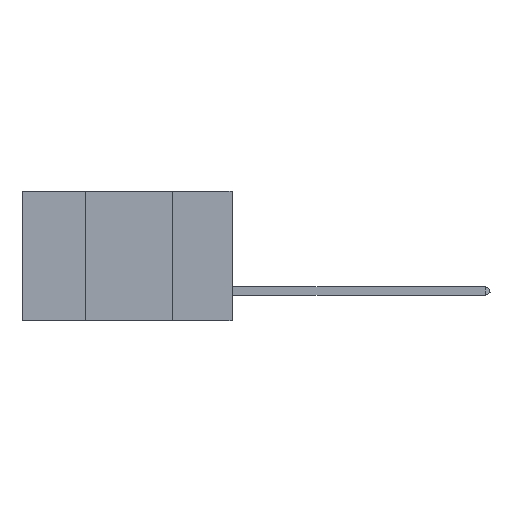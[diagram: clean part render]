
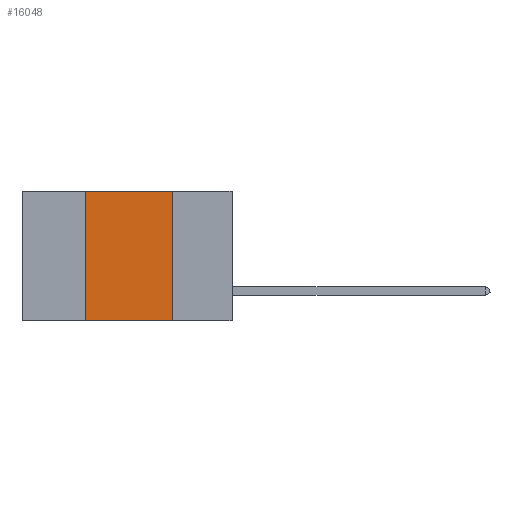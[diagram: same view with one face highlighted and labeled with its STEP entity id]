
A CAD part, left-side view. The second image highlights one B-rep face of the part: STEP entity #16048.
In plain terms, the highlighted planar face has unit normal (-1, 0, 0).
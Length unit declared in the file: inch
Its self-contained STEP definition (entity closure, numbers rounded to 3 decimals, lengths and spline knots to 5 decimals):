
#233 = EDGE_CURVE ( 'NONE', #22224, #1460, #5608, .T. ) ;
#422 = VECTOR ( 'NONE', #11954, 39.37008 ) ;
#1460 = VERTEX_POINT ( 'NONE', #13220 ) ;
#1502 = CARTESIAN_POINT ( 'NONE',  ( 0., 0.6, 0. ) ) ;
#3021 = EDGE_LOOP ( 'NONE', ( #9963, #9471, #19968, #9890 ) ) ;
#3056 = PLANE ( 'NONE',  #6564 ) ;
#3438 = LINE ( 'NONE', #16764, #9142 ) ;
#4448 = EDGE_CURVE ( 'NONE', #4482, #22224, #4647, .T. ) ;
#4482 = VERTEX_POINT ( 'NONE', #10826 ) ;
#4647 = LINE ( 'NONE', #1502, #5725 ) ;
#4759 = CARTESIAN_POINT ( 'NONE',  ( 0., 0.42, -0.37 ) ) ;
#5604 = FACE_OUTER_BOUND ( 'NONE', #3021, .T. ) ;
#5608 = LINE ( 'NONE', #22294, #422 ) ;
#5725 = VECTOR ( 'NONE', #8570, 39.37008 ) ;
#6048 = CARTESIAN_POINT ( 'NONE',  ( 0., 0.17, 0. ) ) ;
#6194 = DIRECTION ( 'NONE',  ( 0., 0., 1. ) ) ;
#6564 = AXIS2_PLACEMENT_3D ( 'NONE', #14696, #7830, #20363 ) ;
#7830 = DIRECTION ( 'NONE',  ( 1., 0., 0. ) ) ;
#8570 = DIRECTION ( 'NONE',  ( 0., -1., 0. ) ) ;
#9142 = VECTOR ( 'NONE', #6194, 39.37008 ) ;
#9471 = ORIENTED_EDGE ( 'NONE', *, *, #4448, .F. ) ;
#9890 = ORIENTED_EDGE ( 'NONE', *, *, #14965, .T. ) ;
#9963 = ORIENTED_EDGE ( 'NONE', *, *, #233, .F. ) ;
#10826 = CARTESIAN_POINT ( 'NONE',  ( 0., 0.42, 0. ) ) ;
#11089 = EDGE_CURVE ( 'NONE', #11139, #4482, #3438, .T. ) ;
#11139 = VERTEX_POINT ( 'NONE', #4759 ) ;
#11954 = DIRECTION ( 'NONE',  ( 0., 0., -1. ) ) ;
#12489 = LINE ( 'NONE', #17504, #20056 ) ;
#13220 = CARTESIAN_POINT ( 'NONE',  ( 0., 0.17, -0.37 ) ) ;
#13827 = DIRECTION ( 'NONE',  ( 0., -1., 0. ) ) ;
#14696 = CARTESIAN_POINT ( 'NONE',  ( 0., 0.6, 0. ) ) ;
#14965 = EDGE_CURVE ( 'NONE', #11139, #1460, #12489, .T. ) ;
#16048 = ADVANCED_FACE ( 'NONE', ( #5604 ), #3056, .F. ) ;
#16764 = CARTESIAN_POINT ( 'NONE',  ( 0., 0.42, 0. ) ) ;
#17504 = CARTESIAN_POINT ( 'NONE',  ( 0., 0.6, -0.37 ) ) ;
#19968 = ORIENTED_EDGE ( 'NONE', *, *, #11089, .F. ) ;
#20056 = VECTOR ( 'NONE', #13827, 39.37008 ) ;
#20363 = DIRECTION ( 'NONE',  ( 0., 0., -1. ) ) ;
#22224 = VERTEX_POINT ( 'NONE', #6048 ) ;
#22294 = CARTESIAN_POINT ( 'NONE',  ( 0., 0.17, 0. ) ) ;
